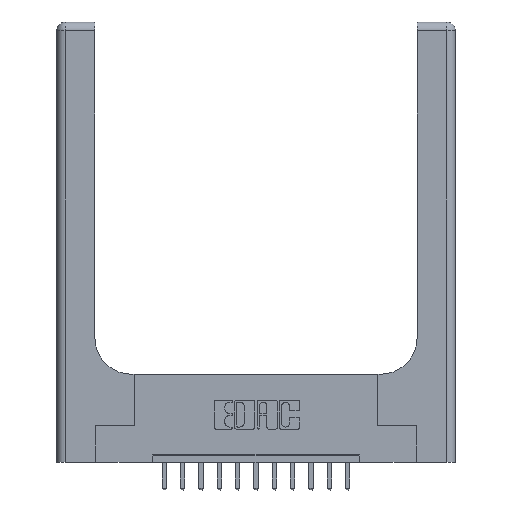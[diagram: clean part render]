
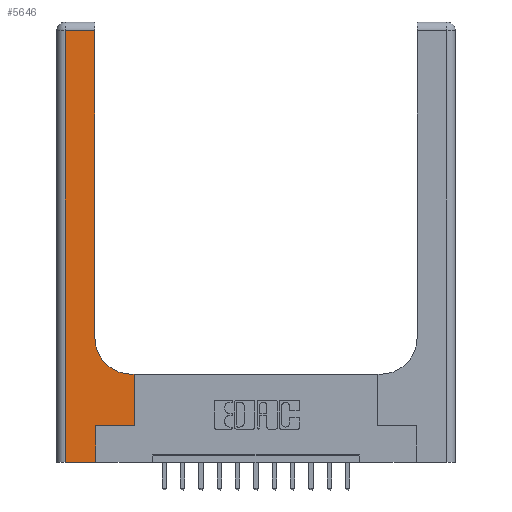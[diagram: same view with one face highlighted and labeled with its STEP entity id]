
A CAD part, top view. The second image highlights one B-rep face of the part: STEP entity #5646.
In plain terms, the highlighted planar face has unit normal (0, 0, 1).
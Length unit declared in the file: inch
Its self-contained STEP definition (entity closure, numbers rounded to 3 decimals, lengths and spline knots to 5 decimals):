
#27 = ORIENTED_EDGE ( 'NONE', *, *, #10505, .T. ) ;
#569 = VECTOR ( 'NONE', #13019, 39.37008 ) ;
#891 = EDGE_CURVE ( 'NONE', #11137, #16688, #6024, .T. ) ;
#1010 = VERTEX_POINT ( 'NONE', #8822 ) ;
#1072 = CARTESIAN_POINT ( 'NONE',  ( 0.26, 3., 0.37 ) ) ;
#1159 = DIRECTION ( 'NONE',  ( 0., -1., 0. ) ) ;
#1447 = LINE ( 'NONE', #2694, #4719 ) ;
#1735 = VECTOR ( 'NONE', #1736, 39.37008 ) ;
#1736 = DIRECTION ( 'NONE',  ( 1., 0., 0. ) ) ;
#1992 = VERTEX_POINT ( 'NONE', #15607 ) ;
#2078 = CARTESIAN_POINT ( 'NONE',  ( 0.265, 0., 0.37 ) ) ;
#2658 = CARTESIAN_POINT ( 'NONE',  ( 0., 2.94, 0.37 ) ) ;
#2694 = CARTESIAN_POINT ( 'NONE',  ( 0.265, 0., 0.37 ) ) ;
#2766 = CIRCLE ( 'NONE', #14128, 0.25 ) ;
#2817 = ORIENTED_EDGE ( 'NONE', *, *, #9094, .T. ) ;
#2823 = CARTESIAN_POINT ( 'NONE',  ( 0., 0., 0.37 ) ) ;
#3443 = ORIENTED_EDGE ( 'NONE', *, *, #9345, .T. ) ;
#4047 = ORIENTED_EDGE ( 'NONE', *, *, #5708, .T. ) ;
#4659 = VERTEX_POINT ( 'NONE', #2078 ) ;
#4719 = VECTOR ( 'NONE', #10422, 39.37008 ) ;
#4850 = CARTESIAN_POINT ( 'NONE',  ( 0.26, 0.6, 0.37 ) ) ;
#4907 = DIRECTION ( 'NONE',  ( 1., 0., 0. ) ) ;
#5100 = CARTESIAN_POINT ( 'NONE',  ( 0.26, 0.85, 0.37 ) ) ;
#5317 = CARTESIAN_POINT ( 'NONE',  ( 0., 3., 0.37 ) ) ;
#5563 = CARTESIAN_POINT ( 'NONE',  ( 0.265, 0.25, 0.37 ) ) ;
#5646 = ADVANCED_FACE ( 'NONE', ( #14281 ), #9302, .F. ) ;
#5708 = EDGE_CURVE ( 'NONE', #7405, #11137, #11669, .T. ) ;
#6024 = LINE ( 'NONE', #12298, #10296 ) ;
#7058 = LINE ( 'NONE', #2658, #569 ) ;
#7068 = VECTOR ( 'NONE', #10030, 39.37008 ) ;
#7251 = AXIS2_PLACEMENT_3D ( 'NONE', #5317, #10398, #8205 ) ;
#7405 = VERTEX_POINT ( 'NONE', #12116 ) ;
#8187 = LINE ( 'NONE', #2823, #1735 ) ;
#8205 = DIRECTION ( 'NONE',  ( -1., 0., 0. ) ) ;
#8561 = EDGE_LOOP ( 'NONE', ( #27, #2817, #9348, #11822, #12345, #4047, #15213, #3443, #10104 ) ) ;
#8728 = VECTOR ( 'NONE', #9034, 39.37008 ) ;
#8822 = CARTESIAN_POINT ( 'NONE',  ( 0.06, 2.94, 0.37 ) ) ;
#9034 = DIRECTION ( 'NONE',  ( 0., 1., 0. ) ) ;
#9094 = EDGE_CURVE ( 'NONE', #11860, #1010, #7058, .T. ) ;
#9302 = PLANE ( 'NONE',  #7251 ) ;
#9345 = EDGE_CURVE ( 'NONE', #16688, #15802, #16430, .T. ) ;
#9348 = ORIENTED_EDGE ( 'NONE', *, *, #15949, .T. ) ;
#9408 = VERTEX_POINT ( 'NONE', #5100 ) ;
#9596 = CARTESIAN_POINT ( 'NONE',  ( 0.528, 0.25, 0.37 ) ) ;
#10004 = CARTESIAN_POINT ( 'NONE',  ( 0.51, 0.85, 0.37 ) ) ;
#10030 = DIRECTION ( 'NONE',  ( -1., 0., 0. ) ) ;
#10104 = ORIENTED_EDGE ( 'NONE', *, *, #12960, .T. ) ;
#10296 = VECTOR ( 'NONE', #11201, 39.37008 ) ;
#10398 = DIRECTION ( 'NONE',  ( 0., 0., -1. ) ) ;
#10422 = DIRECTION ( 'NONE',  ( 0., 1., 0. ) ) ;
#10505 = EDGE_CURVE ( 'NONE', #9408, #11860, #11493, .T. ) ;
#10826 = CARTESIAN_POINT ( 'NONE',  ( 0.26, 2.94, 0.37 ) ) ;
#11137 = VERTEX_POINT ( 'NONE', #9596 ) ;
#11201 = DIRECTION ( 'NONE',  ( 0., 1., 0. ) ) ;
#11493 = LINE ( 'NONE', #1072, #8728 ) ;
#11583 = VECTOR ( 'NONE', #13027, 39.37008 ) ;
#11669 = LINE ( 'NONE', #5563, #11583 ) ;
#11822 = ORIENTED_EDGE ( 'NONE', *, *, #14997, .T. ) ;
#11829 = LINE ( 'NONE', #16709, #13677 ) ;
#11860 = VERTEX_POINT ( 'NONE', #10826 ) ;
#12116 = CARTESIAN_POINT ( 'NONE',  ( 0.265, 0.25, 0.37 ) ) ;
#12298 = CARTESIAN_POINT ( 'NONE',  ( 0.528, 0.25, 0.37 ) ) ;
#12345 = ORIENTED_EDGE ( 'NONE', *, *, #15225, .T. ) ;
#12546 = DIRECTION ( 'NONE',  ( 0., 0., -1. ) ) ;
#12647 = CARTESIAN_POINT ( 'NONE',  ( 0.528, 0.6, 0.37 ) ) ;
#12960 = EDGE_CURVE ( 'NONE', #15802, #9408, #2766, .T. ) ;
#13019 = DIRECTION ( 'NONE',  ( -1., 0., 0. ) ) ;
#13027 = DIRECTION ( 'NONE',  ( 1., 0., 0. ) ) ;
#13677 = VECTOR ( 'NONE', #1159, 39.37008 ) ;
#13943 = CARTESIAN_POINT ( 'NONE',  ( 0.51, 0.6, 0.37 ) ) ;
#14128 = AXIS2_PLACEMENT_3D ( 'NONE', #10004, #12546, #4907 ) ;
#14281 = FACE_OUTER_BOUND ( 'NONE', #8561, .T. ) ;
#14997 = EDGE_CURVE ( 'NONE', #1992, #4659, #8187, .T. ) ;
#15213 = ORIENTED_EDGE ( 'NONE', *, *, #891, .T. ) ;
#15225 = EDGE_CURVE ( 'NONE', #4659, #7405, #1447, .T. ) ;
#15607 = CARTESIAN_POINT ( 'NONE',  ( 0.06, 0., 0.37 ) ) ;
#15802 = VERTEX_POINT ( 'NONE', #13943 ) ;
#15949 = EDGE_CURVE ( 'NONE', #1010, #1992, #11829, .T. ) ;
#16430 = LINE ( 'NONE', #4850, #7068 ) ;
#16688 = VERTEX_POINT ( 'NONE', #12647 ) ;
#16709 = CARTESIAN_POINT ( 'NONE',  ( 0.06, 3., 0.37 ) ) ;
